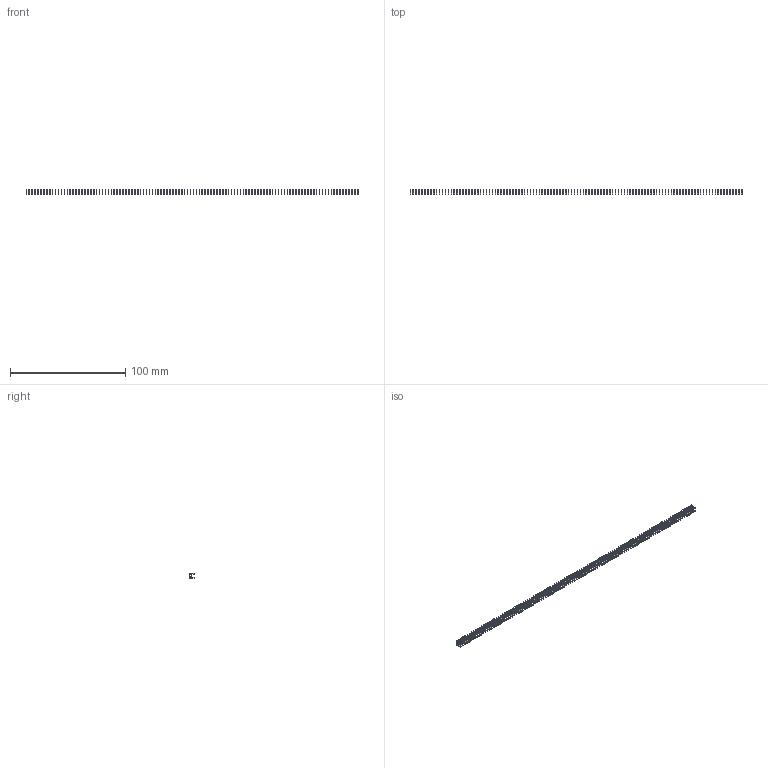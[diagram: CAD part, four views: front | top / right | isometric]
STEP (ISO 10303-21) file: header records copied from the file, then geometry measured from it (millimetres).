
FILE_DESCRIPTION (( 'STEP AP203' ), '1' );
FILE_NAME ('105-114-208-100.STEP', '2020-04-08T01:24:43', ( '' ), ( '' ), 'SwSTEP 2.0', 'SolidWorks 2016', '' );
FILE_SCHEMA (( 'CONFIG_CONTROL_DESIGN' ));
Length unit declared in the file: inch
Products named in the file (2): 100-290-001_100-290-208; 105-114-208-100
Assembly tree (114 placements, depth 2):
  105-114-208-100
    100-290-001_100-290-208  x114
Bounding box: 287.53 x 4.83 x 5.17 mm (x, y, z)
Volume: 784.4 mm3; surface area: 4844.5 mm2
Topology: 114 solids, 114 shells, 2850 faces, 7866 edges, 5244 vertices
Faces by surface type: plane 2508, cylinder 342
Entity records: 4605 total; most frequent: DIRECTION 359, CARTESIAN_POINT 257, CALENDAR_DATE 238, DATE_AND_TIME 238, LOCAL_TIME 238, COORDINATED_UNIVERSAL_TIME_OFFSET 238, AXIS2_PLACEMENT_3D 148, ORIENTED_EDGE 138
